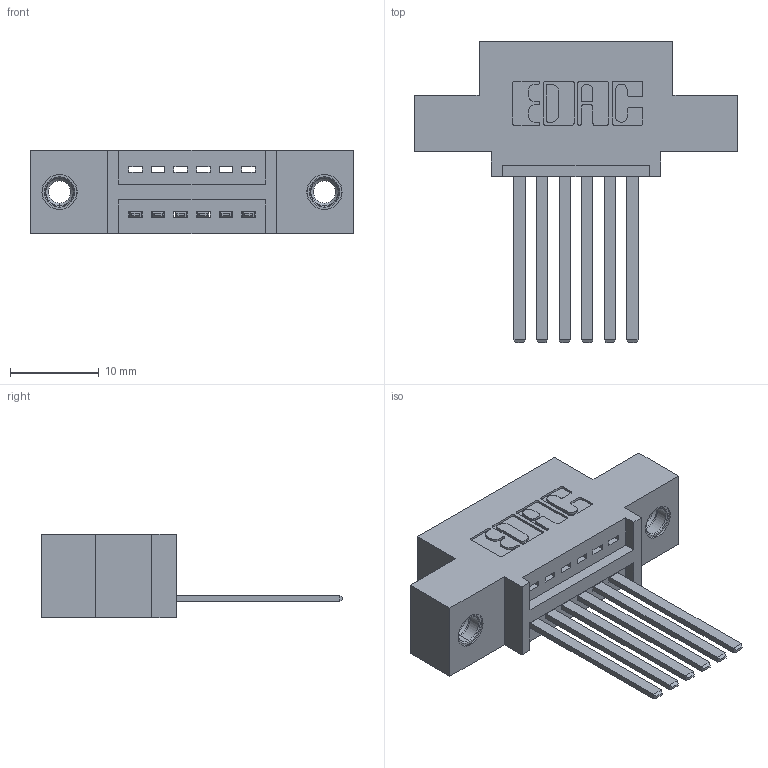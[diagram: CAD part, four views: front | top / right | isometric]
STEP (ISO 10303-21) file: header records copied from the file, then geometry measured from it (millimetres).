
FILE_DESCRIPTION (( 'STEP AP203' ), '1' );
FILE_NAME ('345-006-544-407.STEP', '2019-10-03T16:14:52', ( '' ), ( '' ), 'SwSTEP 2.0', 'SolidWorks 2016', '' );
FILE_SCHEMA (( 'CONFIG_CONTROL_DESIGN' ));
Length unit declared in the file: inch
Products named in the file (4): 345-250-001_345-250-005-103; 345-006-544-407; 345 Part_0.110 Offset - 0.156 Dia-TI; 345-292-001_345-293-144
Assembly tree (9 placements, depth 2):
  345-006-544-407
    345 Part_0.110 Offset - 0.156 Dia-TI
    345-292-001_345-293-144  x6
    345-250-001_345-250-005-103  x2
Bounding box: 36.45 x 33.96 x 9.4 mm (x, y, z)
Volume: 3149.7 mm3; surface area: 4019.4 mm2
Topology: 9 solids, 9 shells, 502 faces, 1437 edges, 942 vertices
Faces by surface type: plane 332, cylinder 154, cone 12, torus 4
Entity records: 10496 total; most frequent: CARTESIAN_POINT 1801, ORIENTED_EDGE 1734, DIRECTION 1649, EDGE_CURVE 867, VECTOR 695, LINE 695, VERTEX_POINT 572, AXIS2_PLACEMENT_3D 477
